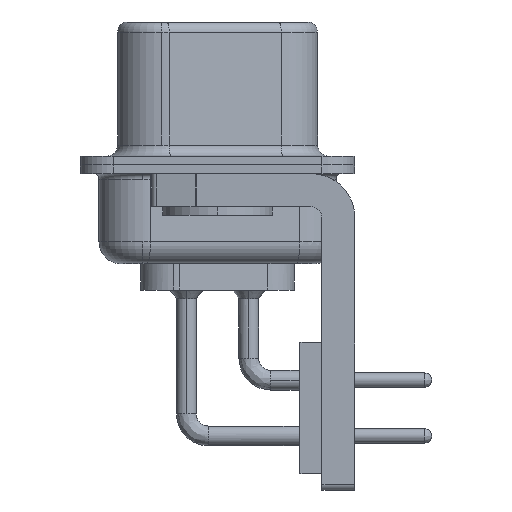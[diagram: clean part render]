
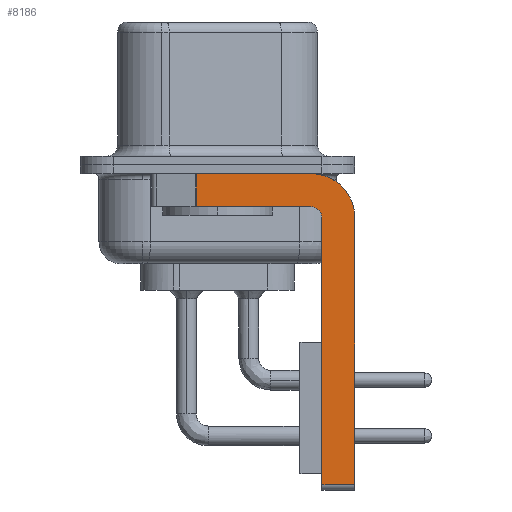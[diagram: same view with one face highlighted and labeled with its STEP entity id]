
A CAD part, left-side view. The second image highlights one B-rep face of the part: STEP entity #8186.
In plain terms, the highlighted planar face has unit normal (-1, 0, 0).
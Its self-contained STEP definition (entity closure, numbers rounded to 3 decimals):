
#169 = AXIS2_PLACEMENT_3D ( 'NONE', #15390, #10993, #26529 ) ;
#213 = CARTESIAN_POINT ( 'NONE',  ( -2.9, -4.25, -0.4 ) ) ;
#349 = EDGE_LOOP ( 'NONE', ( #5094, #2154, #26566, #2855, #27979, #15379, #11041, #26019 ) ) ;
#603 = AXIS2_PLACEMENT_3D ( 'NONE', #10175, #25722, #12441 ) ;
#1283 = VERTEX_POINT ( 'NONE', #4134 ) ;
#1781 = VECTOR ( 'NONE', #2029, 1000. ) ;
#1828 = CARTESIAN_POINT ( 'NONE',  ( -2.9, 0.978, -0.4 ) ) ;
#2029 = DIRECTION ( 'NONE',  ( 0., -1., 0. ) ) ;
#2154 = ORIENTED_EDGE ( 'NONE', *, *, #7565, .T. ) ;
#2855 = ORIENTED_EDGE ( 'NONE', *, *, #18134, .F. ) ;
#2881 = VECTOR ( 'NONE', #11093, 1000. ) ;
#3624 = CARTESIAN_POINT ( 'NONE',  ( -2.9, -6.25, -14.55 ) ) ;
#4134 = CARTESIAN_POINT ( 'NONE',  ( -2.9, -4.25, -1.9 ) ) ;
#4253 = CARTESIAN_POINT ( 'NONE',  ( -2.9, 3., -0.4 ) ) ;
#4269 = PLANE ( 'NONE',  #169 ) ;
#4629 = LINE ( 'NONE', #12659, #28342 ) ;
#5094 = ORIENTED_EDGE ( 'NONE', *, *, #17694, .F. ) ;
#5334 = VERTEX_POINT ( 'NONE', #3624 ) ;
#5959 = DIRECTION ( 'NONE',  ( 1., 0., 0. ) ) ;
#6044 = CARTESIAN_POINT ( 'NONE',  ( -2.9, -4.75, -2.4 ) ) ;
#7565 = EDGE_CURVE ( 'NONE', #12170, #24564, #4629, .T. ) ;
#8186 = ADVANCED_FACE ( 'NONE', ( #18301 ), #4269, .F. ) ;
#8851 = VERTEX_POINT ( 'NONE', #13261 ) ;
#8869 = CARTESIAN_POINT ( 'NONE',  ( -2.9, -6.25, -2.4 ) ) ;
#8921 = LINE ( 'NONE', #20128, #19443 ) ;
#10175 = CARTESIAN_POINT ( 'NONE',  ( -2.9, -4.25, -2.4 ) ) ;
#10317 = CARTESIAN_POINT ( 'NONE',  ( -2.9, -6.25, -2.4 ) ) ;
#10993 = DIRECTION ( 'NONE',  ( 1., 0., 0. ) ) ;
#11041 = ORIENTED_EDGE ( 'NONE', *, *, #20875, .F. ) ;
#11093 = DIRECTION ( 'NONE',  ( 0., 0., -1. ) ) ;
#12047 = VERTEX_POINT ( 'NONE', #10317 ) ;
#12090 = VERTEX_POINT ( 'NONE', #6044 ) ;
#12170 = VERTEX_POINT ( 'NONE', #1828 ) ;
#12441 = DIRECTION ( 'NONE',  ( 0., 0., 1. ) ) ;
#12444 = DIRECTION ( 'NONE',  ( 0., 0., 1. ) ) ;
#12659 = CARTESIAN_POINT ( 'NONE',  ( -2.9, 0.978, -1.9 ) ) ;
#13101 = EDGE_CURVE ( 'NONE', #13411, #12047, #17078, .T. ) ;
#13261 = CARTESIAN_POINT ( 'NONE',  ( -2.9, -4.75, -14.55 ) ) ;
#13411 = VERTEX_POINT ( 'NONE', #213 ) ;
#14441 = LINE ( 'NONE', #4253, #1781 ) ;
#14799 = LINE ( 'NONE', #8869, #2881 ) ;
#15071 = VECTOR ( 'NONE', #21350, 1000. ) ;
#15379 = ORIENTED_EDGE ( 'NONE', *, *, #26557, .T. ) ;
#15390 = CARTESIAN_POINT ( 'NONE',  ( -2.9, -4.25, -2.4 ) ) ;
#17078 = CIRCLE ( 'NONE', #20249, 2. ) ;
#17199 = CIRCLE ( 'NONE', #603, 0.5 ) ;
#17681 = LINE ( 'NONE', #21426, #22860 ) ;
#17694 = EDGE_CURVE ( 'NONE', #12170, #13411, #14441, .T. ) ;
#17986 = DIRECTION ( 'NONE',  ( 0., -1., 0. ) ) ;
#18134 = EDGE_CURVE ( 'NONE', #12090, #1283, #17199, .T. ) ;
#18301 = FACE_OUTER_BOUND ( 'NONE', #349, .T. ) ;
#19157 = CARTESIAN_POINT ( 'NONE',  ( -2.9, -4.25, -1.9 ) ) ;
#19381 = CARTESIAN_POINT ( 'NONE',  ( -2.9, -4.25, -2.4 ) ) ;
#19443 = VECTOR ( 'NONE', #17986, 1000. ) ;
#19448 = CARTESIAN_POINT ( 'NONE',  ( -2.9, 0.978, -1.9 ) ) ;
#20128 = CARTESIAN_POINT ( 'NONE',  ( -2.9, -4.25, -14.55 ) ) ;
#20249 = AXIS2_PLACEMENT_3D ( 'NONE', #19381, #5959, #21564 ) ;
#20875 = EDGE_CURVE ( 'NONE', #12047, #5334, #14799, .T. ) ;
#21350 = DIRECTION ( 'NONE',  ( 0., 1., 0. ) ) ;
#21426 = CARTESIAN_POINT ( 'NONE',  ( -2.9, -4.75, -14.8 ) ) ;
#21564 = DIRECTION ( 'NONE',  ( 0., 0., -1. ) ) ;
#22676 = EDGE_CURVE ( 'NONE', #1283, #24564, #26083, .T. ) ;
#22860 = VECTOR ( 'NONE', #12444, 1000. ) ;
#24564 = VERTEX_POINT ( 'NONE', #19448 ) ;
#25722 = DIRECTION ( 'NONE',  ( -1., 0., 0. ) ) ;
#26019 = ORIENTED_EDGE ( 'NONE', *, *, #13101, .F. ) ;
#26083 = LINE ( 'NONE', #19157, #15071 ) ;
#26529 = DIRECTION ( 'NONE',  ( 0., 0., -1. ) ) ;
#26557 = EDGE_CURVE ( 'NONE', #8851, #5334, #8921, .T. ) ;
#26566 = ORIENTED_EDGE ( 'NONE', *, *, #22676, .F. ) ;
#26927 = EDGE_CURVE ( 'NONE', #8851, #12090, #17681, .T. ) ;
#27979 = ORIENTED_EDGE ( 'NONE', *, *, #26927, .F. ) ;
#28185 = DIRECTION ( 'NONE',  ( 0., 0., -1. ) ) ;
#28342 = VECTOR ( 'NONE', #28185, 1000. ) ;
